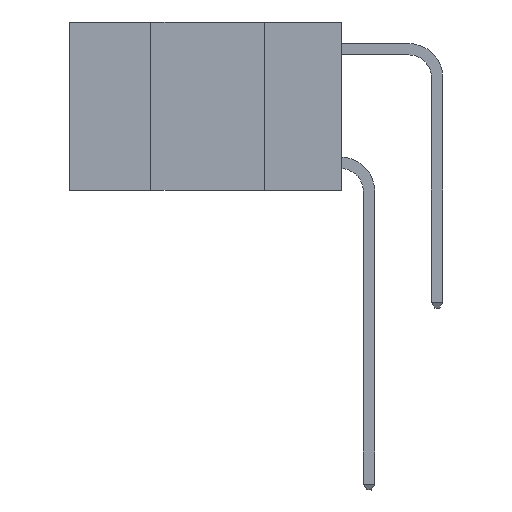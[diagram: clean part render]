
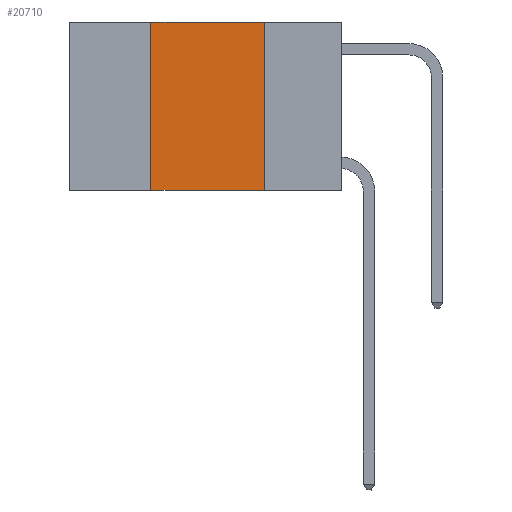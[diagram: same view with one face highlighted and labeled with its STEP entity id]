
A CAD part, left-side view. The second image highlights one B-rep face of the part: STEP entity #20710.
In plain terms, the highlighted planar face has unit normal (-1, 0, 0).
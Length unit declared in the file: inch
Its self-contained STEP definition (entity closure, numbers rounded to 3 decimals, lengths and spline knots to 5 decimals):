
#121 = CARTESIAN_POINT ( 'NONE',  ( 0., 0.6, 0. ) ) ;
#1162 = ORIENTED_EDGE ( 'NONE', *, *, #14835, .F. ) ;
#2077 = VERTEX_POINT ( 'NONE', #20684 ) ;
#3552 = VECTOR ( 'NONE', #23455, 39.37008 ) ;
#4285 = EDGE_CURVE ( 'NONE', #7814, #2077, #21429, .T. ) ;
#5651 = LINE ( 'NONE', #26113, #14335 ) ;
#6184 = DIRECTION ( 'NONE',  ( 0., 0., -1. ) ) ;
#6576 = CARTESIAN_POINT ( 'NONE',  ( 0., 0.42, 0. ) ) ;
#6625 = CARTESIAN_POINT ( 'NONE',  ( 0., 0.17, 0. ) ) ;
#7119 = ORIENTED_EDGE ( 'NONE', *, *, #4285, .F. ) ;
#7307 = CARTESIAN_POINT ( 'NONE',  ( 0., 0.17, 0. ) ) ;
#7814 = VERTEX_POINT ( 'NONE', #19666 ) ;
#7919 = VERTEX_POINT ( 'NONE', #7307 ) ;
#8121 = VERTEX_POINT ( 'NONE', #21609 ) ;
#8640 = AXIS2_PLACEMENT_3D ( 'NONE', #27096, #18820, #6184 ) ;
#11797 = LINE ( 'NONE', #121, #17382 ) ;
#13633 = DIRECTION ( 'NONE',  ( 0., -1., 0. ) ) ;
#14335 = VECTOR ( 'NONE', #13633, 39.37008 ) ;
#14835 = EDGE_CURVE ( 'NONE', #7919, #8121, #19766, .T. ) ;
#15853 = VECTOR ( 'NONE', #23322, 39.37008 ) ;
#16055 = ORIENTED_EDGE ( 'NONE', *, *, #16104, .F. ) ;
#16104 = EDGE_CURVE ( 'NONE', #2077, #7919, #11797, .T. ) ;
#17382 = VECTOR ( 'NONE', #23302, 39.37008 ) ;
#18221 = EDGE_LOOP ( 'NONE', ( #1162, #16055, #7119, #18707 ) ) ;
#18707 = ORIENTED_EDGE ( 'NONE', *, *, #21723, .T. ) ;
#18820 = DIRECTION ( 'NONE',  ( 1., 0., 0. ) ) ;
#19666 = CARTESIAN_POINT ( 'NONE',  ( 0., 0.42, -0.37 ) ) ;
#19766 = LINE ( 'NONE', #6625, #3552 ) ;
#20684 = CARTESIAN_POINT ( 'NONE',  ( 0., 0.42, 0. ) ) ;
#20710 = ADVANCED_FACE ( 'NONE', ( #26271 ), #22846, .F. ) ;
#21429 = LINE ( 'NONE', #6576, #15853 ) ;
#21609 = CARTESIAN_POINT ( 'NONE',  ( 0., 0.17, -0.37 ) ) ;
#21723 = EDGE_CURVE ( 'NONE', #7814, #8121, #5651, .T. ) ;
#22846 = PLANE ( 'NONE',  #8640 ) ;
#23302 = DIRECTION ( 'NONE',  ( 0., -1., 0. ) ) ;
#23322 = DIRECTION ( 'NONE',  ( 0., 0., 1. ) ) ;
#23455 = DIRECTION ( 'NONE',  ( 0., 0., -1. ) ) ;
#26113 = CARTESIAN_POINT ( 'NONE',  ( 0., 0.6, -0.37 ) ) ;
#26271 = FACE_OUTER_BOUND ( 'NONE', #18221, .T. ) ;
#27096 = CARTESIAN_POINT ( 'NONE',  ( 0., 0.6, 0. ) ) ;
